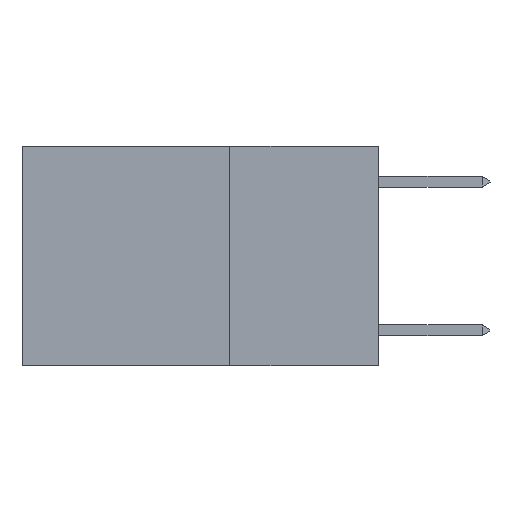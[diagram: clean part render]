
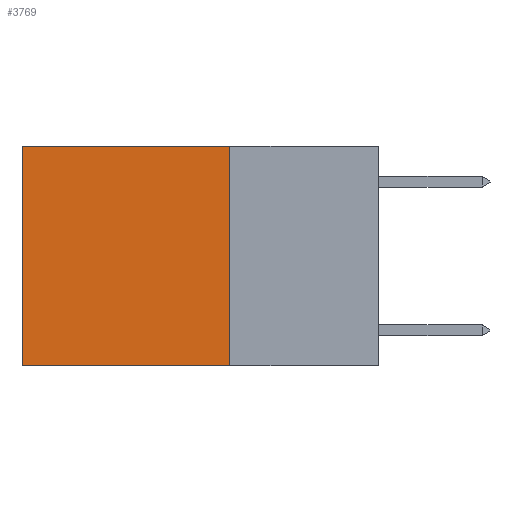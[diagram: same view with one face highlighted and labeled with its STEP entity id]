
A CAD part, left-side view. The second image highlights one B-rep face of the part: STEP entity #3769.
In plain terms, the highlighted planar face has unit normal (-1, 0, 0).
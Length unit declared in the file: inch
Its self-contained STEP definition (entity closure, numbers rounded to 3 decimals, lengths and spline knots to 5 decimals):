
#317 = CARTESIAN_POINT ( 'NONE',  ( 0.2625, 0.6, 0. ) ) ;
#411 = FACE_OUTER_BOUND ( 'NONE', #6035, .T. ) ;
#588 = VECTOR ( 'NONE', #9572, 39.37008 ) ;
#990 = EDGE_CURVE ( 'NONE', #7939, #4490, #8635, .T. ) ;
#1065 = PLANE ( 'NONE',  #5699 ) ;
#1323 = CARTESIAN_POINT ( 'NONE',  ( 0.2625, 0.6, -0.37 ) ) ;
#1719 = DIRECTION ( 'NONE',  ( 0., 0., -1. ) ) ;
#2025 = ORIENTED_EDGE ( 'NONE', *, *, #990, .F. ) ;
#2573 = CARTESIAN_POINT ( 'NONE',  ( 0.2625, 0.25, 0. ) ) ;
#2711 = LINE ( 'NONE', #7744, #588 ) ;
#2857 = DIRECTION ( 'NONE',  ( 0., 0., -1. ) ) ;
#3769 = ADVANCED_FACE ( 'NONE', ( #411 ), #1065, .F. ) ;
#4189 = LINE ( 'NONE', #2573, #10837 ) ;
#4367 = DIRECTION ( 'NONE',  ( 0., 1., 0. ) ) ;
#4490 = VERTEX_POINT ( 'NONE', #1323 ) ;
#4570 = CARTESIAN_POINT ( 'NONE',  ( 0.2625, 0.6, 0. ) ) ;
#4607 = CARTESIAN_POINT ( 'NONE',  ( 0.2625, 0.25, -0.37 ) ) ;
#5441 = DIRECTION ( 'NONE',  ( 0., 0., -1. ) ) ;
#5699 = AXIS2_PLACEMENT_3D ( 'NONE', #8096, #7863, #5441 ) ;
#5993 = EDGE_CURVE ( 'NONE', #10327, #7939, #4189, .T. ) ;
#6035 = EDGE_LOOP ( 'NONE', ( #7261, #2025, #7496, #9893 ) ) ;
#6242 = LINE ( 'NONE', #317, #9790 ) ;
#6637 = EDGE_CURVE ( 'NONE', #6895, #4490, #6242, .T. ) ;
#6680 = VECTOR ( 'NONE', #4367, 39.37008 ) ;
#6895 = VERTEX_POINT ( 'NONE', #4570 ) ;
#7261 = ORIENTED_EDGE ( 'NONE', *, *, #6637, .T. ) ;
#7496 = ORIENTED_EDGE ( 'NONE', *, *, #5993, .F. ) ;
#7744 = CARTESIAN_POINT ( 'NONE',  ( 0.2625, 0.25, 0. ) ) ;
#7863 = DIRECTION ( 'NONE',  ( 1., 0., 0. ) ) ;
#7939 = VERTEX_POINT ( 'NONE', #11126 ) ;
#8096 = CARTESIAN_POINT ( 'NONE',  ( 0.2625, 0.25, 0. ) ) ;
#8289 = CARTESIAN_POINT ( 'NONE',  ( 0.2625, 0.25, 0. ) ) ;
#8539 = EDGE_CURVE ( 'NONE', #10327, #6895, #2711, .T. ) ;
#8635 = LINE ( 'NONE', #4607, #6680 ) ;
#9572 = DIRECTION ( 'NONE',  ( 0., 1., 0. ) ) ;
#9790 = VECTOR ( 'NONE', #2857, 39.37008 ) ;
#9893 = ORIENTED_EDGE ( 'NONE', *, *, #8539, .T. ) ;
#10327 = VERTEX_POINT ( 'NONE', #8289 ) ;
#10837 = VECTOR ( 'NONE', #1719, 39.37008 ) ;
#11126 = CARTESIAN_POINT ( 'NONE',  ( 0.2625, 0.25, -0.37 ) ) ;
